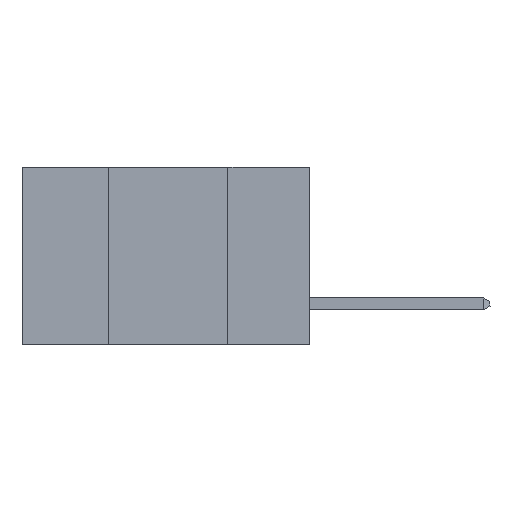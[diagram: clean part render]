
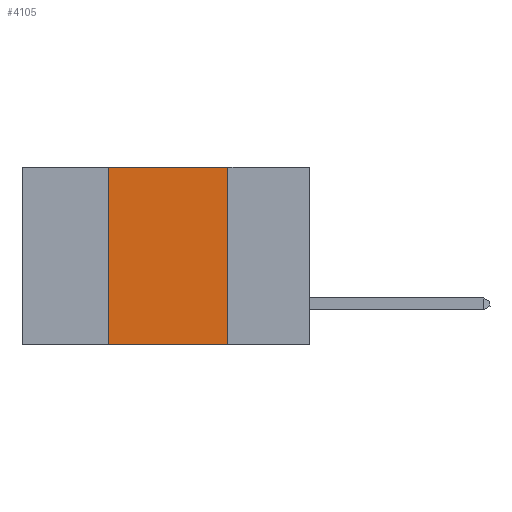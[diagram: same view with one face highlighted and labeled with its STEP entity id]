
A CAD part, left-side view. The second image highlights one B-rep face of the part: STEP entity #4105.
In plain terms, the highlighted planar face has unit normal (-1, 0, 0).
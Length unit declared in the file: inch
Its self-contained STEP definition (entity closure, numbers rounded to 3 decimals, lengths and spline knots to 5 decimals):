
#2096 = DIRECTION ( 'NONE',  ( 0., 0., -1. ) ) ;
#2143 = DIRECTION ( 'NONE',  ( 1., 0., 0. ) ) ;
#2303 = PLANE ( 'NONE',  #13250 ) ;
#2533 = CARTESIAN_POINT ( 'NONE',  ( 0., 0.6, 0. ) ) ;
#2609 = EDGE_CURVE ( 'NONE', #17142, #12930, #16938, .T. ) ;
#3291 = EDGE_CURVE ( 'NONE', #11612, #3914, #3484, .T. ) ;
#3484 = LINE ( 'NONE', #14117, #7241 ) ;
#3640 = CARTESIAN_POINT ( 'NONE',  ( 0., 0.42, 0. ) ) ;
#3914 = VERTEX_POINT ( 'NONE', #4940 ) ;
#3965 = LINE ( 'NONE', #3640, #11926 ) ;
#4105 = ADVANCED_FACE ( 'NONE', ( #5259 ), #2303, .F. ) ;
#4334 = ORIENTED_EDGE ( 'NONE', *, *, #6496, .F. ) ;
#4369 = EDGE_CURVE ( 'NONE', #11612, #17142, #3965, .T. ) ;
#4802 = CARTESIAN_POINT ( 'NONE',  ( 0., 0.17, 0. ) ) ;
#4940 = CARTESIAN_POINT ( 'NONE',  ( 0., 0.17, -0.37 ) ) ;
#5259 = FACE_OUTER_BOUND ( 'NONE', #6841, .T. ) ;
#5288 = DIRECTION ( 'NONE',  ( 0., 0., 1. ) ) ;
#6496 = EDGE_CURVE ( 'NONE', #12930, #3914, #18786, .T. ) ;
#6841 = EDGE_LOOP ( 'NONE', ( #4334, #12568, #12282, #12322 ) ) ;
#7241 = VECTOR ( 'NONE', #14447, 39.37008 ) ;
#9599 = CARTESIAN_POINT ( 'NONE',  ( 0., 0.42, -0.37 ) ) ;
#10711 = CARTESIAN_POINT ( 'NONE',  ( 0., 0.42, 0. ) ) ;
#11612 = VERTEX_POINT ( 'NONE', #9599 ) ;
#11825 = VECTOR ( 'NONE', #13994, 39.37008 ) ;
#11926 = VECTOR ( 'NONE', #5288, 39.37008 ) ;
#12282 = ORIENTED_EDGE ( 'NONE', *, *, #4369, .F. ) ;
#12322 = ORIENTED_EDGE ( 'NONE', *, *, #3291, .T. ) ;
#12424 = CARTESIAN_POINT ( 'NONE',  ( 0., 0.17, 0. ) ) ;
#12568 = ORIENTED_EDGE ( 'NONE', *, *, #2609, .F. ) ;
#12930 = VERTEX_POINT ( 'NONE', #4802 ) ;
#13250 = AXIS2_PLACEMENT_3D ( 'NONE', #2533, #2143, #2096 ) ;
#13994 = DIRECTION ( 'NONE',  ( 0., 0., -1. ) ) ;
#14117 = CARTESIAN_POINT ( 'NONE',  ( 0., 0.6, -0.37 ) ) ;
#14310 = CARTESIAN_POINT ( 'NONE',  ( 0., 0.6, 0. ) ) ;
#14447 = DIRECTION ( 'NONE',  ( 0., -1., 0. ) ) ;
#14559 = DIRECTION ( 'NONE',  ( 0., -1., 0. ) ) ;
#16938 = LINE ( 'NONE', #14310, #20601 ) ;
#17142 = VERTEX_POINT ( 'NONE', #10711 ) ;
#18786 = LINE ( 'NONE', #12424, #11825 ) ;
#20601 = VECTOR ( 'NONE', #14559, 39.37008 ) ;
